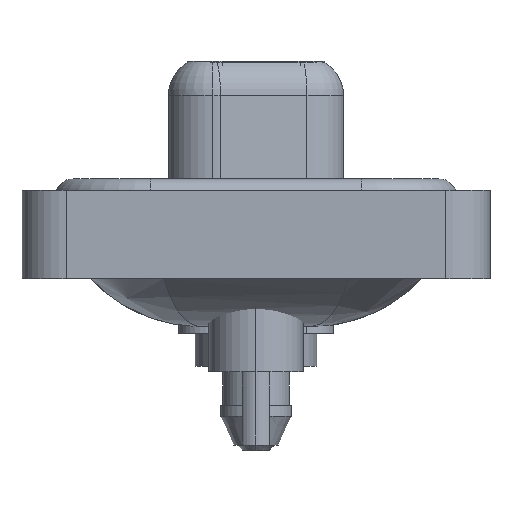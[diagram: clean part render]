
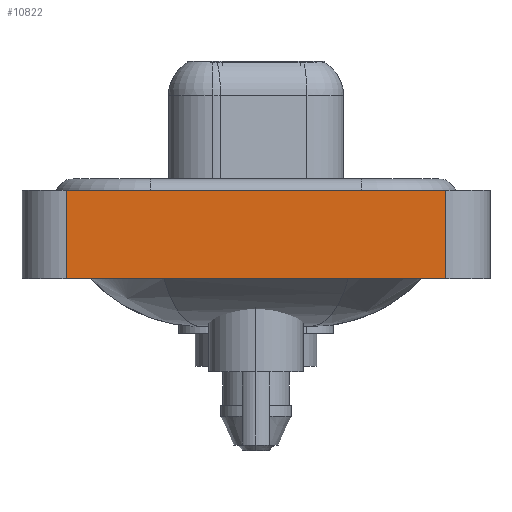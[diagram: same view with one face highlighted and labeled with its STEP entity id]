
A CAD part, left-side view. The second image highlights one B-rep face of the part: STEP entity #10822.
In plain terms, the highlighted planar face has unit normal (-1, 0, 0).
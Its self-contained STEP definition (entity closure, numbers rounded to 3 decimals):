
#216 = CARTESIAN_POINT ( 'NONE',  ( -7.3, -8.55, -3.6 ) ) ;
#754 = VECTOR ( 'NONE', #1226, 1000. ) ;
#1226 = DIRECTION ( 'NONE',  ( 0., 0., 1. ) ) ;
#1719 = ORIENTED_EDGE ( 'NONE', *, *, #4667, .F. ) ;
#1934 = ORIENTED_EDGE ( 'NONE', *, *, #14416, .T. ) ;
#2273 = VERTEX_POINT ( 'NONE', #15805 ) ;
#2388 = LINE ( 'NONE', #4068, #754 ) ;
#2585 = AXIS2_PLACEMENT_3D ( 'NONE', #8098, #5348, #9274 ) ;
#3029 = VERTEX_POINT ( 'NONE', #7948 ) ;
#3652 = VECTOR ( 'NONE', #13652, 1000. ) ;
#4068 = CARTESIAN_POINT ( 'NONE',  ( -7.3, -8.55, -3.6 ) ) ;
#4170 = VERTEX_POINT ( 'NONE', #8947 ) ;
#4243 = ORIENTED_EDGE ( 'NONE', *, *, #10576, .T. ) ;
#4667 = EDGE_CURVE ( 'NONE', #2273, #4170, #11791, .T. ) ;
#5133 = EDGE_LOOP ( 'NONE', ( #1934, #1719, #17211, #4243 ) ) ;
#5162 = FACE_OUTER_BOUND ( 'NONE', #5133, .T. ) ;
#5348 = DIRECTION ( 'NONE',  ( -1., 0., 0. ) ) ;
#6403 = DIRECTION ( 'NONE',  ( 0., -1., 0. ) ) ;
#7948 = CARTESIAN_POINT ( 'NONE',  ( -7.3, 8.55, -3.6 ) ) ;
#8098 = CARTESIAN_POINT ( 'NONE',  ( -7.3, -8.55, -3.6 ) ) ;
#8131 = VECTOR ( 'NONE', #17092, 1000. ) ;
#8947 = CARTESIAN_POINT ( 'NONE',  ( -7.3, -8.55, 0.4 ) ) ;
#9274 = DIRECTION ( 'NONE',  ( 0., 0., 1. ) ) ;
#9302 = LINE ( 'NONE', #16286, #3652 ) ;
#10565 = VECTOR ( 'NONE', #6403, 1000. ) ;
#10576 = EDGE_CURVE ( 'NONE', #3029, #12988, #17179, .T. ) ;
#10822 = ADVANCED_FACE ( 'NONE', ( #5162 ), #13278, .T. ) ;
#11791 = LINE ( 'NONE', #14518, #8131 ) ;
#12988 = VERTEX_POINT ( 'NONE', #216 ) ;
#13102 = CARTESIAN_POINT ( 'NONE',  ( -7.3, -8.55, -3.6 ) ) ;
#13278 = PLANE ( 'NONE',  #2585 ) ;
#13652 = DIRECTION ( 'NONE',  ( 0., 0., 1. ) ) ;
#14416 = EDGE_CURVE ( 'NONE', #12988, #4170, #2388, .T. ) ;
#14518 = CARTESIAN_POINT ( 'NONE',  ( -7.3, -8.55, 0.4 ) ) ;
#15805 = CARTESIAN_POINT ( 'NONE',  ( -7.3, 8.55, 0.4 ) ) ;
#16286 = CARTESIAN_POINT ( 'NONE',  ( -7.3, 8.55, -3.6 ) ) ;
#17092 = DIRECTION ( 'NONE',  ( 0., -1., 0. ) ) ;
#17179 = LINE ( 'NONE', #13102, #10565 ) ;
#17211 = ORIENTED_EDGE ( 'NONE', *, *, #17482, .F. ) ;
#17482 = EDGE_CURVE ( 'NONE', #3029, #2273, #9302, .T. ) ;
